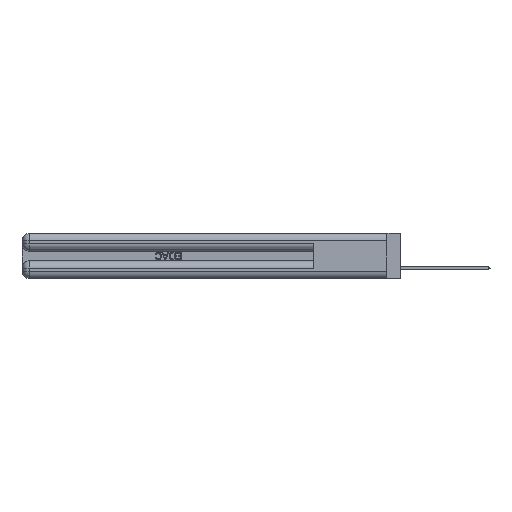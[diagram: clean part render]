
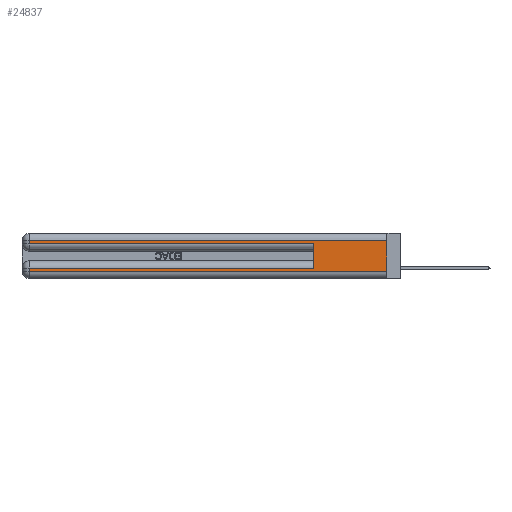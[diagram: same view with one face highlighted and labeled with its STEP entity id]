
A CAD part, left-side view. The second image highlights one B-rep face of the part: STEP entity #24837.
In plain terms, the highlighted planar face has unit normal (-1, 0, 0).
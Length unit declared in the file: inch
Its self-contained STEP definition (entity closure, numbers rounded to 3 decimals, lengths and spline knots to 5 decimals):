
#1638 = VECTOR ( 'NONE', #8537, 39.37008 ) ;
#1653 = ORIENTED_EDGE ( 'NONE', *, *, #7283, .T. ) ;
#1657 = EDGE_CURVE ( 'NONE', #35816, #31229, #20559, .T. ) ;
#2337 = EDGE_LOOP ( 'NONE', ( #5017, #44097, #16552, #29137, #31141, #41846, #1653, #38107 ) ) ;
#4553 = CARTESIAN_POINT ( 'NONE',  ( 0., 0., 0.31 ) ) ;
#5017 = ORIENTED_EDGE ( 'NONE', *, *, #25354, .F. ) ;
#5027 = CARTESIAN_POINT ( 'NONE',  ( 0., 0., 0.06 ) ) ;
#6137 = LINE ( 'NONE', #37733, #7727 ) ;
#6322 = EDGE_CURVE ( 'NONE', #11790, #39077, #29903, .T. ) ;
#6610 = CARTESIAN_POINT ( 'NONE',  ( 0., 2.94, 0.06 ) ) ;
#7283 = EDGE_CURVE ( 'NONE', #13034, #28928, #39012, .T. ) ;
#7727 = VECTOR ( 'NONE', #13333, 39.37008 ) ;
#8242 = CARTESIAN_POINT ( 'NONE',  ( 0., 0., 0.285 ) ) ;
#8537 = DIRECTION ( 'NONE',  ( 0., -1., 0. ) ) ;
#8683 = DIRECTION ( 'NONE',  ( 0., -1., 0. ) ) ;
#10044 = VECTOR ( 'NONE', #11384, 39.37008 ) ;
#10379 = VECTOR ( 'NONE', #15485, 39.37008 ) ;
#10488 = EDGE_CURVE ( 'NONE', #39077, #28316, #36948, .T. ) ;
#11090 = CARTESIAN_POINT ( 'NONE',  ( 0., 0., 0.37 ) ) ;
#11331 = VECTOR ( 'NONE', #19225, 39.37008 ) ;
#11384 = DIRECTION ( 'NONE',  ( 0., 0., -1. ) ) ;
#11790 = VERTEX_POINT ( 'NONE', #44721 ) ;
#13034 = VERTEX_POINT ( 'NONE', #38475 ) ;
#13333 = DIRECTION ( 'NONE',  ( 0., 1., 0. ) ) ;
#14315 = CARTESIAN_POINT ( 'NONE',  ( 0., 0.6, 0.085 ) ) ;
#14399 = DIRECTION ( 'NONE',  ( 1., 0., 0. ) ) ;
#14406 = CARTESIAN_POINT ( 'NONE',  ( 0., 2.94, 0.31 ) ) ;
#14542 = DIRECTION ( 'NONE',  ( 0., 0., -1. ) ) ;
#14694 = LINE ( 'NONE', #5027, #1638 ) ;
#15485 = DIRECTION ( 'NONE',  ( 0., 1., 0. ) ) ;
#16552 = ORIENTED_EDGE ( 'NONE', *, *, #10488, .T. ) ;
#17918 = PLANE ( 'NONE',  #36936 ) ;
#17983 = EDGE_CURVE ( 'NONE', #35816, #13034, #6137, .T. ) ;
#19225 = DIRECTION ( 'NONE',  ( 0., 0., 1. ) ) ;
#20141 = CARTESIAN_POINT ( 'NONE',  ( 0., 2.94, 0.37 ) ) ;
#20559 = LINE ( 'NONE', #38796, #11331 ) ;
#23556 = EDGE_CURVE ( 'NONE', #28316, #31229, #25437, .T. ) ;
#24586 = CARTESIAN_POINT ( 'NONE',  ( 0., 0., 0.06 ) ) ;
#24837 = ADVANCED_FACE ( 'NONE', ( #44249 ), #17918, .F. ) ;
#25354 = EDGE_CURVE ( 'NONE', #11790, #26941, #27964, .T. ) ;
#25437 = LINE ( 'NONE', #8242, #27623 ) ;
#26941 = VERTEX_POINT ( 'NONE', #24586 ) ;
#27623 = VECTOR ( 'NONE', #8683, 39.37008 ) ;
#27743 = VECTOR ( 'NONE', #38632, 39.37008 ) ;
#27964 = LINE ( 'NONE', #32489, #10044 ) ;
#28316 = VERTEX_POINT ( 'NONE', #33716 ) ;
#28928 = VERTEX_POINT ( 'NONE', #6610 ) ;
#29137 = ORIENTED_EDGE ( 'NONE', *, *, #23556, .T. ) ;
#29903 = LINE ( 'NONE', #4553, #10379 ) ;
#31141 = ORIENTED_EDGE ( 'NONE', *, *, #1657, .F. ) ;
#31229 = VERTEX_POINT ( 'NONE', #39343 ) ;
#31449 = VECTOR ( 'NONE', #40882, 39.37008 ) ;
#32489 = CARTESIAN_POINT ( 'NONE',  ( 0., 0., 0.37 ) ) ;
#33716 = CARTESIAN_POINT ( 'NONE',  ( 0., 2.94, 0.285 ) ) ;
#34210 = EDGE_CURVE ( 'NONE', #28928, #26941, #14694, .T. ) ;
#35816 = VERTEX_POINT ( 'NONE', #14315 ) ;
#36936 = AXIS2_PLACEMENT_3D ( 'NONE', #11090, #14399, #14542 ) ;
#36948 = LINE ( 'NONE', #38344, #27743 ) ;
#37733 = CARTESIAN_POINT ( 'NONE',  ( 0., 0., 0.085 ) ) ;
#38107 = ORIENTED_EDGE ( 'NONE', *, *, #34210, .T. ) ;
#38344 = CARTESIAN_POINT ( 'NONE',  ( 0., 2.94, 0.37 ) ) ;
#38475 = CARTESIAN_POINT ( 'NONE',  ( 0., 2.94, 0.085 ) ) ;
#38632 = DIRECTION ( 'NONE',  ( 0., 0., -1. ) ) ;
#38796 = CARTESIAN_POINT ( 'NONE',  ( 0., 0.6, 0.145 ) ) ;
#39012 = LINE ( 'NONE', #20141, #31449 ) ;
#39077 = VERTEX_POINT ( 'NONE', #14406 ) ;
#39343 = CARTESIAN_POINT ( 'NONE',  ( 0., 0.6, 0.285 ) ) ;
#40882 = DIRECTION ( 'NONE',  ( 0., 0., -1. ) ) ;
#41846 = ORIENTED_EDGE ( 'NONE', *, *, #17983, .T. ) ;
#44097 = ORIENTED_EDGE ( 'NONE', *, *, #6322, .T. ) ;
#44249 = FACE_OUTER_BOUND ( 'NONE', #2337, .T. ) ;
#44721 = CARTESIAN_POINT ( 'NONE',  ( 0., 0., 0.31 ) ) ;
